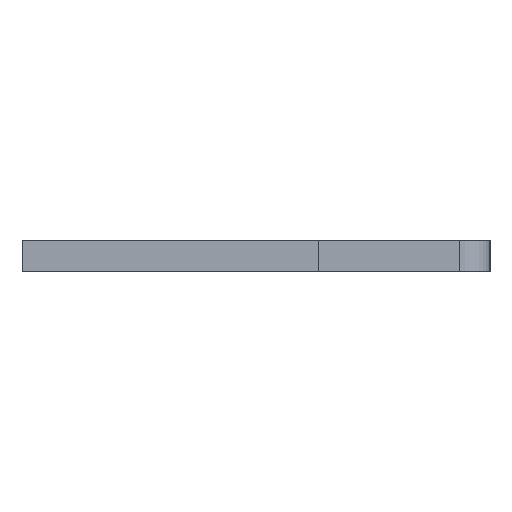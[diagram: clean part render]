
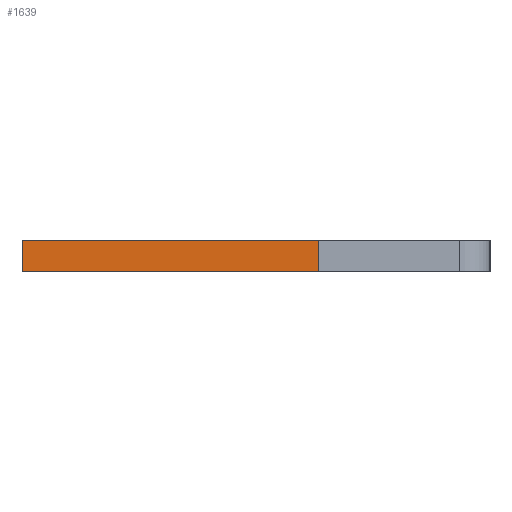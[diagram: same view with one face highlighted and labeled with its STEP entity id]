
A CAD part, left-side view. The second image highlights one B-rep face of the part: STEP entity #1639.
In plain terms, the highlighted face is planar.
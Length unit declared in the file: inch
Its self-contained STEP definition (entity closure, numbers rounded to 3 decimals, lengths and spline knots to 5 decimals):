
#26 = EDGE_LOOP ( 'NONE', ( #1226, #1650, #1020, #85 ) ) ;
#62 = DIRECTION ( 'NONE',  ( 0., 0., 1. ) ) ;
#82 = LINE ( 'NONE', #517, #1937 ) ;
#85 = ORIENTED_EDGE ( 'NONE', *, *, #566, .T. ) ;
#113 = DIRECTION ( 'NONE',  ( -1., 0., 0. ) ) ;
#160 = VECTOR ( 'NONE', #1543, 39.37008 ) ;
#169 = EDGE_CURVE ( 'NONE', #1742, #934, #1123, .T. ) ;
#484 = AXIS2_PLACEMENT_3D ( 'NONE', #1004, #62, #1143 ) ;
#517 = CARTESIAN_POINT ( 'NONE',  ( -0.01, 0.15, -0.04 ) ) ;
#519 = VERTEX_POINT ( 'NONE', #1046 ) ;
#566 = EDGE_CURVE ( 'NONE', #1742, #519, #1873, .T. ) ;
#657 = LINE ( 'NONE', #1234, #160 ) ;
#719 = EDGE_CURVE ( 'NONE', #934, #1263, #657, .T. ) ;
#798 = CARTESIAN_POINT ( 'NONE',  ( -0.01, 0.15, -0.04 ) ) ;
#844 = DIRECTION ( 'NONE',  ( 0., 1., 0. ) ) ;
#934 = VERTEX_POINT ( 'NONE', #944 ) ;
#944 = CARTESIAN_POINT ( 'NONE',  ( 0.01, 0.15, -0.04 ) ) ;
#994 = PLANE ( 'NONE',  #484 ) ;
#1004 = CARTESIAN_POINT ( 'NONE',  ( 0.01, 0.15, -0.04 ) ) ;
#1020 = ORIENTED_EDGE ( 'NONE', *, *, #169, .F. ) ;
#1042 = CARTESIAN_POINT ( 'NONE',  ( 0.01, -0.04, -0.04 ) ) ;
#1046 = CARTESIAN_POINT ( 'NONE',  ( -0.01, -0.04, -0.04 ) ) ;
#1123 = LINE ( 'NONE', #1208, #1740 ) ;
#1143 = DIRECTION ( 'NONE',  ( 1., 0., 0. ) ) ;
#1172 = FACE_OUTER_BOUND ( 'NONE', #26, .T. ) ;
#1208 = CARTESIAN_POINT ( 'NONE',  ( 0.01, 0.15, -0.04 ) ) ;
#1226 = ORIENTED_EDGE ( 'NONE', *, *, #1610, .T. ) ;
#1234 = CARTESIAN_POINT ( 'NONE',  ( 0.01, 0.15, -0.04 ) ) ;
#1263 = VERTEX_POINT ( 'NONE', #798 ) ;
#1359 = DIRECTION ( 'NONE',  ( 0., 1., 0. ) ) ;
#1514 = CARTESIAN_POINT ( 'NONE',  ( 0.01, -0.04, -0.04 ) ) ;
#1543 = DIRECTION ( 'NONE',  ( -1., 0., 0. ) ) ;
#1564 = VECTOR ( 'NONE', #113, 39.37008 ) ;
#1610 = EDGE_CURVE ( 'NONE', #519, #1263, #82, .T. ) ;
#1639 = ADVANCED_FACE ( 'NONE', ( #1172 ), #994, .F. ) ;
#1650 = ORIENTED_EDGE ( 'NONE', *, *, #719, .F. ) ;
#1740 = VECTOR ( 'NONE', #1359, 39.37008 ) ;
#1742 = VERTEX_POINT ( 'NONE', #1514 ) ;
#1873 = LINE ( 'NONE', #1042, #1564 ) ;
#1937 = VECTOR ( 'NONE', #844, 39.37008 ) ;
